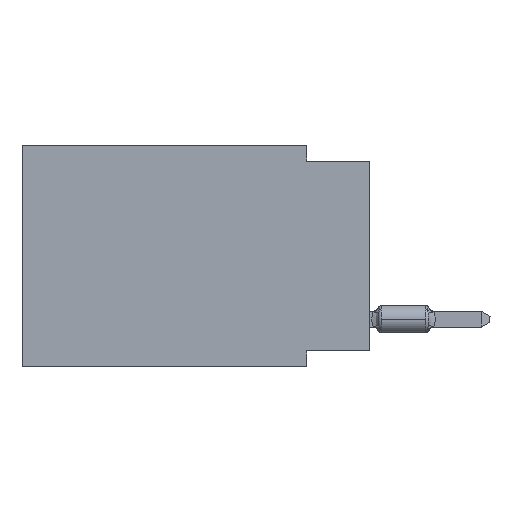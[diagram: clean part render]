
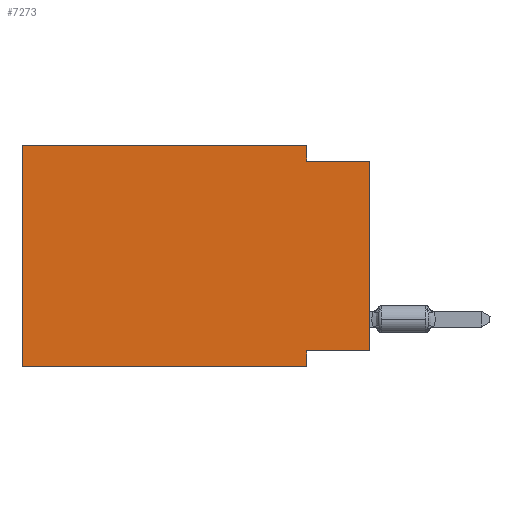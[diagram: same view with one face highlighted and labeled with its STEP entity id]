
A CAD part, left-side view. The second image highlights one B-rep face of the part: STEP entity #7273.
In plain terms, the highlighted planar face has unit normal (-1, 0, 0).
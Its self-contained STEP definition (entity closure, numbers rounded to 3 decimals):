
#681 = CARTESIAN_POINT ( 'NONE',  ( 0., 2.54, -8.89 ) ) ;
#720 = VECTOR ( 'NONE', #21354, 1000. ) ;
#927 = VERTEX_POINT ( 'NONE', #8112 ) ;
#1338 = ORIENTED_EDGE ( 'NONE', *, *, #28706, .T. ) ;
#2612 = ORIENTED_EDGE ( 'NONE', *, *, #18900, .F. ) ;
#2760 = VERTEX_POINT ( 'NONE', #25323 ) ;
#2909 = CARTESIAN_POINT ( 'NONE',  ( 0., 13.97, 0. ) ) ;
#3081 = DIRECTION ( 'NONE',  ( 1., 0., 0. ) ) ;
#4575 = CARTESIAN_POINT ( 'NONE',  ( 0., 13.97, 0. ) ) ;
#4598 = EDGE_CURVE ( 'NONE', #20242, #38294, #40786, .T. ) ;
#5177 = EDGE_LOOP ( 'NONE', ( #38435, #2612, #16482, #28168, #15009, #1338, #40638, #37363 ) ) ;
#5532 = VERTEX_POINT ( 'NONE', #21479 ) ;
#5873 = CARTESIAN_POINT ( 'NONE',  ( 0., 2.54, -8.89 ) ) ;
#6716 = PLANE ( 'NONE',  #14545 ) ;
#6849 = VERTEX_POINT ( 'NONE', #5873 ) ;
#7273 = ADVANCED_FACE ( 'NONE', ( #34768 ), #6716, .F. ) ;
#8112 = CARTESIAN_POINT ( 'NONE',  ( 0., 2.54, 0. ) ) ;
#8192 = DIRECTION ( 'NONE',  ( 0., 0., -1. ) ) ;
#8945 = LINE ( 'NONE', #22638, #31195 ) ;
#9887 = VECTOR ( 'NONE', #42972, 1000. ) ;
#11513 = DIRECTION ( 'NONE',  ( 0., 0., -1. ) ) ;
#12509 = VECTOR ( 'NONE', #11513, 1000. ) ;
#13378 = LINE ( 'NONE', #27278, #16213 ) ;
#14030 = DIRECTION ( 'NONE',  ( 0., 0., -1. ) ) ;
#14213 = EDGE_CURVE ( 'NONE', #927, #2760, #42998, .T. ) ;
#14545 = AXIS2_PLACEMENT_3D ( 'NONE', #4575, #3081, #14030 ) ;
#15009 = ORIENTED_EDGE ( 'NONE', *, *, #4598, .F. ) ;
#16213 = VECTOR ( 'NONE', #30029, 1000. ) ;
#16482 = ORIENTED_EDGE ( 'NONE', *, *, #14213, .F. ) ;
#17331 = CARTESIAN_POINT ( 'NONE',  ( 0., 2.54, -8.255 ) ) ;
#18111 = VECTOR ( 'NONE', #8192, 1000. ) ;
#18900 = EDGE_CURVE ( 'NONE', #2760, #32031, #34946, .T. ) ;
#19163 = CARTESIAN_POINT ( 'NONE',  ( 0., 13.97, 0. ) ) ;
#19381 = CARTESIAN_POINT ( 'NONE',  ( 0., 0., -0.635 ) ) ;
#20242 = VERTEX_POINT ( 'NONE', #21720 ) ;
#21354 = DIRECTION ( 'NONE',  ( 0., -1., 0. ) ) ;
#21479 = CARTESIAN_POINT ( 'NONE',  ( 0., 0., -8.255 ) ) ;
#21720 = CARTESIAN_POINT ( 'NONE',  ( 0., 13.97, -8.89 ) ) ;
#22215 = EDGE_CURVE ( 'NONE', #5532, #41484, #37841, .T. ) ;
#22321 = VECTOR ( 'NONE', #30743, 1000. ) ;
#22638 = CARTESIAN_POINT ( 'NONE',  ( 0., 0., 0. ) ) ;
#24141 = CARTESIAN_POINT ( 'NONE',  ( 0., 0., -8.255 ) ) ;
#25092 = VECTOR ( 'NONE', #28546, 1000. ) ;
#25323 = CARTESIAN_POINT ( 'NONE',  ( 0., 2.54, -0.635 ) ) ;
#26115 = CARTESIAN_POINT ( 'NONE',  ( 0., 2.54, 0. ) ) ;
#27278 = CARTESIAN_POINT ( 'NONE',  ( 0., 13.97, 0. ) ) ;
#28168 = ORIENTED_EDGE ( 'NONE', *, *, #31263, .F. ) ;
#28423 = LINE ( 'NONE', #29093, #720 ) ;
#28546 = DIRECTION ( 'NONE',  ( 0., -1., 0. ) ) ;
#28706 = EDGE_CURVE ( 'NONE', #20242, #6849, #28423, .T. ) ;
#29093 = CARTESIAN_POINT ( 'NONE',  ( 0., 13.97, -8.89 ) ) ;
#30029 = DIRECTION ( 'NONE',  ( 0., -1., 0. ) ) ;
#30743 = DIRECTION ( 'NONE',  ( 0., 0., 1. ) ) ;
#31195 = VECTOR ( 'NONE', #36999, 1000. ) ;
#31263 = EDGE_CURVE ( 'NONE', #38294, #927, #13378, .T. ) ;
#31743 = CARTESIAN_POINT ( 'NONE',  ( 0., 0., -0.635 ) ) ;
#32031 = VERTEX_POINT ( 'NONE', #19381 ) ;
#34768 = FACE_OUTER_BOUND ( 'NONE', #5177, .T. ) ;
#34946 = LINE ( 'NONE', #31743, #25092 ) ;
#36999 = DIRECTION ( 'NONE',  ( 0., 0., 1. ) ) ;
#37363 = ORIENTED_EDGE ( 'NONE', *, *, #22215, .F. ) ;
#37841 = LINE ( 'NONE', #24141, #9887 ) ;
#38294 = VERTEX_POINT ( 'NONE', #19163 ) ;
#38435 = ORIENTED_EDGE ( 'NONE', *, *, #41555, .T. ) ;
#39454 = LINE ( 'NONE', #681, #18111 ) ;
#40638 = ORIENTED_EDGE ( 'NONE', *, *, #41852, .F. ) ;
#40786 = LINE ( 'NONE', #2909, #22321 ) ;
#41484 = VERTEX_POINT ( 'NONE', #17331 ) ;
#41555 = EDGE_CURVE ( 'NONE', #5532, #32031, #8945, .T. ) ;
#41852 = EDGE_CURVE ( 'NONE', #41484, #6849, #39454, .T. ) ;
#42972 = DIRECTION ( 'NONE',  ( 0., 1., 0. ) ) ;
#42998 = LINE ( 'NONE', #26115, #12509 ) ;
